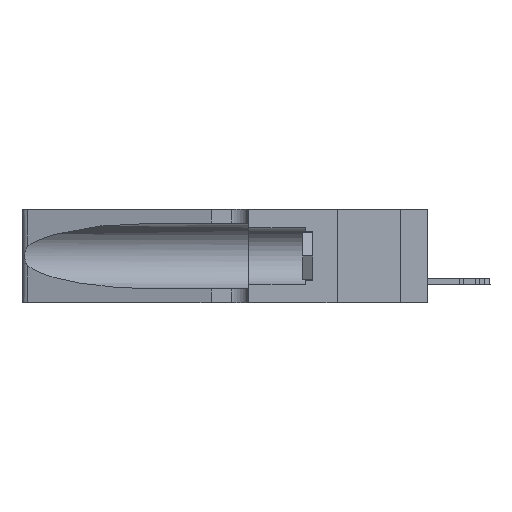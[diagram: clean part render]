
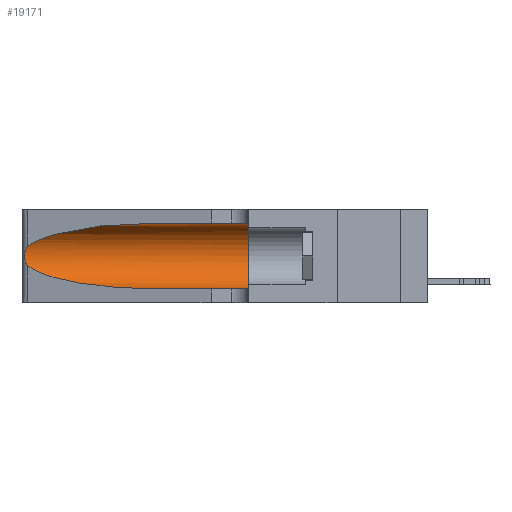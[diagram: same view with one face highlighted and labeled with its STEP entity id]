
A CAD part, left-side view. The second image highlights one B-rep face of the part: STEP entity #19171.
In plain terms, the highlighted cylindrical face has radius 3.308 mm (diameter 6.617 mm), a partial arc.
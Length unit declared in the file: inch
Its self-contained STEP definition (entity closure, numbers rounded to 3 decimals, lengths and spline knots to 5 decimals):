
#1469 = CIRCLE ( 'NONE', #21163, 0.13025 ) ;
#2913 = CARTESIAN_POINT ( 'NONE',  ( 0.26017, 1.23833, 0.17102 ) ) ;
#4026 = VERTEX_POINT ( 'NONE', #41956 ) ;
#4304 = VERTEX_POINT ( 'NONE', #20696 ) ;
#4823 = DIRECTION ( 'NONE',  ( 0., -1., 0. ) ) ;
#5502 = EDGE_LOOP ( 'NONE', ( #5515, #15137, #7907, #12769, #26210, #16850 ) ) ;
#5515 = ORIENTED_EDGE ( 'NONE', *, *, #28736, .T. ) ;
#6752 = VECTOR ( 'NONE', #17281, 39.37008 ) ;
#6945 = AXIS2_PLACEMENT_3D ( 'NONE', #15929, #23756, #29609 ) ;
#7545 = CARTESIAN_POINT ( 'NONE',  ( 0.2373, 1.15595, 0.28018 ) ) ;
#7790 = LINE ( 'NONE', #9845, #6752 ) ;
#7907 = ORIENTED_EDGE ( 'NONE', *, *, #24657, .T. ) ;
#9562 = CARTESIAN_POINT ( 'NONE',  ( 0.25639, 1.23186, 0.15144 ) ) ;
#9845 = CARTESIAN_POINT ( 'NONE',  ( 0.1305, 1.61858, 0.05475 ) ) ;
#9881 = CARTESIAN_POINT ( 'NONE',  ( 0.18966, 0.96281, 0.05475 ) ) ;
#12730 = VERTEX_POINT ( 'NONE', #26262 ) ;
#12769 = ORIENTED_EDGE ( 'NONE', *, *, #32081, .T. ) ;
#13376 = CARTESIAN_POINT ( 'NONE',  ( 0.25487, 1.22718, 0.14631 ) ) ;
#14438 = EDGE_CURVE ( 'NONE', #12730, #4026, #27435, .T. ) ;
#15065 = EDGE_CURVE ( 'NONE', #37939, #28851, #32388, .T. ) ;
#15137 = ORIENTED_EDGE ( 'NONE', *, *, #14438, .T. ) ;
#15441 =( BOUNDED_CURVE ( )  B_SPLINE_CURVE ( 3, ( #43652, #36674, #7545, #22286 ),
 .UNSPECIFIED., .F., .F. ) 
 B_SPLINE_CURVE_WITH_KNOTS ( ( 4, 4 ),
 ( 1.5708, 2.84003 ),
 .UNSPECIFIED. ) 
 CURVE ( )  GEOMETRIC_REPRESENTATION_ITEM ( )  RATIONAL_B_SPLINE_CURVE ( ( 1., 0.87, 0.87, 1. ) ) 
 REPRESENTATION_ITEM ( '' )  );
#15929 = CARTESIAN_POINT ( 'NONE',  ( 0.1305, 1.61858, 0.185 ) ) ;
#16850 = ORIENTED_EDGE ( 'NONE', *, *, #15065, .F. ) ;
#17281 = DIRECTION ( 'NONE',  ( 0., -1., 0. ) ) ;
#18217 = EDGE_CURVE ( 'NONE', #28851, #42011, #1469, .T. ) ;
#19171 = ADVANCED_FACE ( 'NONE', ( #19454 ), #34839, .F. ) ;
#19454 = FACE_OUTER_BOUND ( 'NONE', #5502, .T. ) ;
#20696 = CARTESIAN_POINT ( 'NONE',  ( 0.1305, 0.72297, 0.05475 ) ) ;
#21163 = AXIS2_PLACEMENT_3D ( 'NONE', #31724, #26253, #30031 ) ;
#22286 = CARTESIAN_POINT ( 'NONE',  ( 0.25487, 1.22718, 0.22369 ) ) ;
#23756 = DIRECTION ( 'NONE',  ( 0., -1., 0. ) ) ;
#24610 = CARTESIAN_POINT ( 'NONE',  ( 0.26075, 1.23896, 0.178 ) ) ;
#24657 = EDGE_CURVE ( 'NONE', #4026, #4304, #32364, .T. ) ;
#25553 = CARTESIAN_POINT ( 'NONE',  ( 0.2373, 1.15595, 0.08982 ) ) ;
#26210 = ORIENTED_EDGE ( 'NONE', *, *, #18217, .F. ) ;
#26253 = DIRECTION ( 'NONE',  ( 0., 1., 0. ) ) ;
#26262 = CARTESIAN_POINT ( 'NONE',  ( 0.25487, 1.22718, 0.22369 ) ) ;
#26409 = CARTESIAN_POINT ( 'NONE',  ( 0.1305, 1.61858, 0.31525 ) ) ;
#27435 = B_SPLINE_CURVE_WITH_KNOTS ( 'NONE', 3,
 ( #34798, #36563, #40643, #33020, #35493, #46552, #41002, #24610, #2913, #34305, #42628, #9562, #34916, #13376 ),
 .UNSPECIFIED., .F., .F.,
 ( 4, 2, 2, 2, 2, 2, 4 ),
 ( 0., 0.00027, 0.00053, 0.00107, 0.0016, 0.00187, 0.00214 ),
 .UNSPECIFIED. ) ;
#28445 = VECTOR ( 'NONE', #4823, 39.37008 ) ;
#28736 = EDGE_CURVE ( 'NONE', #37939, #12730, #15441, .T. ) ;
#28851 = VERTEX_POINT ( 'NONE', #31976 ) ;
#29609 = DIRECTION ( 'NONE',  ( 0., 0., -1. ) ) ;
#30031 = DIRECTION ( 'NONE',  ( 0., 0., 1. ) ) ;
#31724 = CARTESIAN_POINT ( 'NONE',  ( 0.1305, 0.35, 0.185 ) ) ;
#31976 = CARTESIAN_POINT ( 'NONE',  ( 0.1305, 0.35, 0.31525 ) ) ;
#32081 = EDGE_CURVE ( 'NONE', #4304, #42011, #7790, .T. ) ;
#32364 =( BOUNDED_CURVE ( )  B_SPLINE_CURVE ( 3, ( #35077, #25553, #9881, #38963 ),
 .UNSPECIFIED., .F., .F. ) 
 B_SPLINE_CURVE_WITH_KNOTS ( ( 4, 4 ),
 ( 3.44316, 4.71239 ),
 .UNSPECIFIED. ) 
 CURVE ( )  GEOMETRIC_REPRESENTATION_ITEM ( )  RATIONAL_B_SPLINE_CURVE ( ( 1., 0.87, 0.87, 1. ) ) 
 REPRESENTATION_ITEM ( '' )  );
#32388 = LINE ( 'NONE', #26409, #28445 ) ;
#33020 = CARTESIAN_POINT ( 'NONE',  ( 0.25787, 1.23484, 0.2124 ) ) ;
#34167 = CARTESIAN_POINT ( 'NONE',  ( 0.1305, 0.72297, 0.31525 ) ) ;
#34305 = CARTESIAN_POINT ( 'NONE',  ( 0.25856, 1.23593, 0.16098 ) ) ;
#34798 = CARTESIAN_POINT ( 'NONE',  ( 0.25487, 1.22718, 0.22369 ) ) ;
#34839 = CYLINDRICAL_SURFACE ( 'NONE', #6945, 0.13025 ) ;
#34916 = CARTESIAN_POINT ( 'NONE',  ( 0.25555, 1.22993, 0.14849 ) ) ;
#35077 = CARTESIAN_POINT ( 'NONE',  ( 0.25487, 1.22718, 0.14631 ) ) ;
#35493 = CARTESIAN_POINT ( 'NONE',  ( 0.25854, 1.2359, 0.20912 ) ) ;
#36563 = CARTESIAN_POINT ( 'NONE',  ( 0.25555, 1.22994, 0.2215 ) ) ;
#36674 = CARTESIAN_POINT ( 'NONE',  ( 0.18966, 0.96281, 0.31525 ) ) ;
#37939 = VERTEX_POINT ( 'NONE', #34167 ) ;
#38963 = CARTESIAN_POINT ( 'NONE',  ( 0.1305, 0.72297, 0.05475 ) ) ;
#40643 = CARTESIAN_POINT ( 'NONE',  ( 0.25639, 1.23184, 0.21858 ) ) ;
#41002 = CARTESIAN_POINT ( 'NONE',  ( 0.26075, 1.23896, 0.19203 ) ) ;
#41956 = CARTESIAN_POINT ( 'NONE',  ( 0.25487, 1.22718, 0.14631 ) ) ;
#42011 = VERTEX_POINT ( 'NONE', #45970 ) ;
#42628 = CARTESIAN_POINT ( 'NONE',  ( 0.25789, 1.23486, 0.15765 ) ) ;
#43652 = CARTESIAN_POINT ( 'NONE',  ( 0.1305, 0.72297, 0.31525 ) ) ;
#45970 = CARTESIAN_POINT ( 'NONE',  ( 0.1305, 0.35, 0.05475 ) ) ;
#46552 = CARTESIAN_POINT ( 'NONE',  ( 0.26018, 1.23835, 0.19895 ) ) ;
